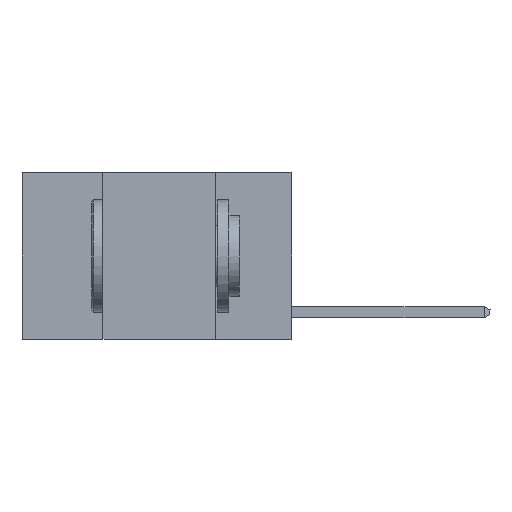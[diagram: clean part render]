
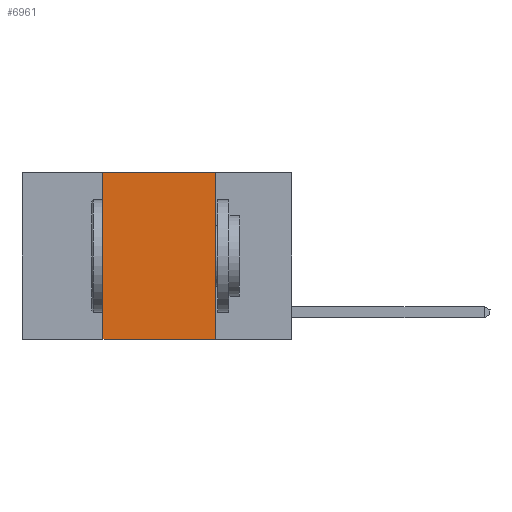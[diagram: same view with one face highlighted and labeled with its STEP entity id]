
A CAD part, left-side view. The second image highlights one B-rep face of the part: STEP entity #6961.
In plain terms, the highlighted planar face has unit normal (-1, 0, 0).
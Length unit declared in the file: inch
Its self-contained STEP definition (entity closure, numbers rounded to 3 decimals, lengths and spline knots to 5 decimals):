
#497 = LINE ( 'NONE', #11503, #8730 ) ;
#652 = CARTESIAN_POINT ( 'NONE',  ( 0., 0.6, 0. ) ) ;
#1069 = VERTEX_POINT ( 'NONE', #13350 ) ;
#1146 = DIRECTION ( 'NONE',  ( 0., 0., 1. ) ) ;
#1677 = EDGE_LOOP ( 'NONE', ( #9019, #9135, #11722, #3716 ) ) ;
#2037 = VERTEX_POINT ( 'NONE', #9253 ) ;
#2275 = CARTESIAN_POINT ( 'NONE',  ( 0., 0.17, 0. ) ) ;
#2809 = DIRECTION ( 'NONE',  ( 0., 0., -1. ) ) ;
#3613 = FACE_OUTER_BOUND ( 'NONE', #1677, .T. ) ;
#3716 = ORIENTED_EDGE ( 'NONE', *, *, #4953, .T. ) ;
#4953 = EDGE_CURVE ( 'NONE', #7825, #10364, #497, .T. ) ;
#5485 = DIRECTION ( 'NONE',  ( 0., 0., -1. ) ) ;
#5624 = VECTOR ( 'NONE', #5485, 39.37008 ) ;
#6147 = DIRECTION ( 'NONE',  ( 0., -1., 0. ) ) ;
#6326 = EDGE_CURVE ( 'NONE', #7825, #1069, #10544, .T. ) ;
#6487 = CARTESIAN_POINT ( 'NONE',  ( 0., 0.42, 0. ) ) ;
#6618 = CARTESIAN_POINT ( 'NONE',  ( 0., 0.6, 0. ) ) ;
#6937 = CARTESIAN_POINT ( 'NONE',  ( 0., 0.17, -0.37 ) ) ;
#6961 = ADVANCED_FACE ( 'NONE', ( #3613 ), #8145, .F. ) ;
#7699 = DIRECTION ( 'NONE',  ( 0., -1., 0. ) ) ;
#7777 = EDGE_CURVE ( 'NONE', #2037, #10364, #8469, .T. ) ;
#7825 = VERTEX_POINT ( 'NONE', #13004 ) ;
#7987 = VECTOR ( 'NONE', #1146, 39.37008 ) ;
#8145 = PLANE ( 'NONE',  #12756 ) ;
#8469 = LINE ( 'NONE', #2275, #5624 ) ;
#8730 = VECTOR ( 'NONE', #6147, 39.37008 ) ;
#9019 = ORIENTED_EDGE ( 'NONE', *, *, #7777, .F. ) ;
#9135 = ORIENTED_EDGE ( 'NONE', *, *, #13357, .F. ) ;
#9253 = CARTESIAN_POINT ( 'NONE',  ( 0., 0.17, 0. ) ) ;
#9263 = DIRECTION ( 'NONE',  ( 1., 0., 0. ) ) ;
#10364 = VERTEX_POINT ( 'NONE', #6937 ) ;
#10544 = LINE ( 'NONE', #6487, #7987 ) ;
#11052 = VECTOR ( 'NONE', #7699, 39.37008 ) ;
#11373 = LINE ( 'NONE', #6618, #11052 ) ;
#11503 = CARTESIAN_POINT ( 'NONE',  ( 0., 0.6, -0.37 ) ) ;
#11722 = ORIENTED_EDGE ( 'NONE', *, *, #6326, .F. ) ;
#12756 = AXIS2_PLACEMENT_3D ( 'NONE', #652, #9263, #2809 ) ;
#13004 = CARTESIAN_POINT ( 'NONE',  ( 0., 0.42, -0.37 ) ) ;
#13350 = CARTESIAN_POINT ( 'NONE',  ( 0., 0.42, 0. ) ) ;
#13357 = EDGE_CURVE ( 'NONE', #1069, #2037, #11373, .T. ) ;
